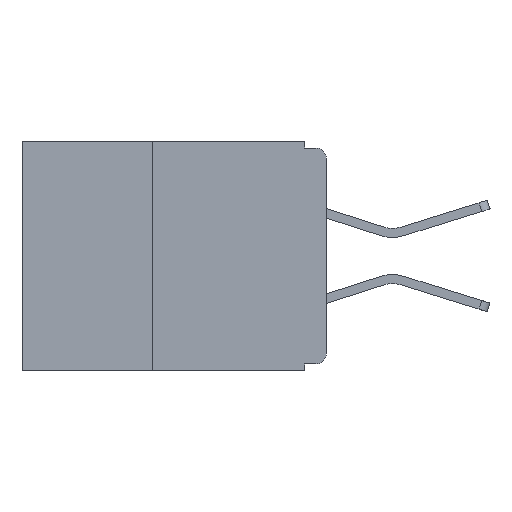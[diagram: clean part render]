
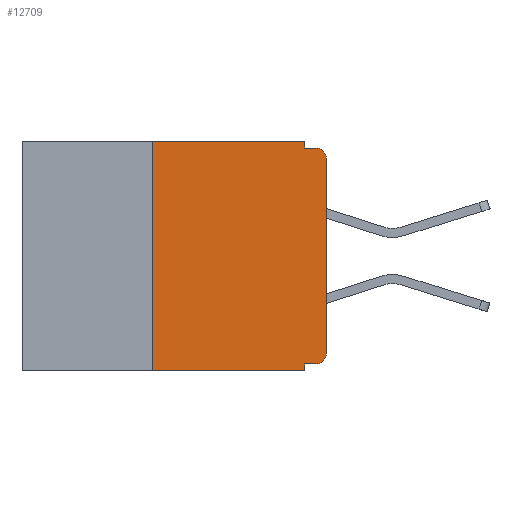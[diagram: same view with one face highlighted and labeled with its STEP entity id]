
A CAD part, left-side view. The second image highlights one B-rep face of the part: STEP entity #12709.
In plain terms, the highlighted planar face has unit normal (-1, 0, 0).
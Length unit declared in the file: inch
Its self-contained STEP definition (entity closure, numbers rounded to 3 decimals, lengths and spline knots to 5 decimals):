
#767 = DIRECTION ( 'NONE',  ( 0., -1., 0. ) ) ;
#1368 = ORIENTED_EDGE ( 'NONE', *, *, #15920, .T. ) ;
#1962 = ORIENTED_EDGE ( 'NONE', *, *, #22748, .T. ) ;
#2030 = LINE ( 'NONE', #27527, #7602 ) ;
#2207 = CARTESIAN_POINT ( 'NONE',  ( 0., 0., -0.305 ) ) ;
#3035 = VERTEX_POINT ( 'NONE', #9136 ) ;
#3124 = VERTEX_POINT ( 'NONE', #2207 ) ;
#3830 = ORIENTED_EDGE ( 'NONE', *, *, #6988, .F. ) ;
#3945 = CARTESIAN_POINT ( 'NONE',  ( 0., 0.031, 0. ) ) ;
#6203 = CARTESIAN_POINT ( 'NONE',  ( 0., 0.015, -0.025 ) ) ;
#6988 = EDGE_CURVE ( 'NONE', #7017, #12612, #12422, .T. ) ;
#7017 = VERTEX_POINT ( 'NONE', #26400 ) ;
#7403 = CARTESIAN_POINT ( 'NONE',  ( 0., 0., -0.025 ) ) ;
#7602 = VECTOR ( 'NONE', #25388, 39.37008 ) ;
#8556 = DIRECTION ( 'NONE',  ( 0., 0., -1. ) ) ;
#8704 = DIRECTION ( 'NONE',  ( 0., 0., -1. ) ) ;
#9136 = CARTESIAN_POINT ( 'NONE',  ( 0., 0.25, -0.33 ) ) ;
#9165 = DIRECTION ( 'NONE',  ( 0., -1., 0. ) ) ;
#9817 = CIRCLE ( 'NONE', #23273, 0.015 ) ;
#10277 = CARTESIAN_POINT ( 'NONE',  ( 0., 0.437, -0.33 ) ) ;
#10391 = CARTESIAN_POINT ( 'NONE',  ( 0., 0.031, -0.32 ) ) ;
#10599 = VERTEX_POINT ( 'NONE', #28992 ) ;
#10800 = CARTESIAN_POINT ( 'NONE',  ( 0., 0.25, -0.33 ) ) ;
#10866 = DIRECTION ( 'NONE',  ( 0., -1., 0. ) ) ;
#10928 = AXIS2_PLACEMENT_3D ( 'NONE', #6203, #22020, #8556 ) ;
#11355 = EDGE_CURVE ( 'NONE', #7017, #3124, #9817, .T. ) ;
#11557 = LINE ( 'NONE', #10800, #12267 ) ;
#11936 = LINE ( 'NONE', #29159, #28253 ) ;
#12267 = VECTOR ( 'NONE', #22029, 39.37008 ) ;
#12422 = LINE ( 'NONE', #27696, #29430 ) ;
#12612 = VERTEX_POINT ( 'NONE', #10391 ) ;
#12709 = ADVANCED_FACE ( 'NONE', ( #18882 ), #17483, .F. ) ;
#12977 = CARTESIAN_POINT ( 'NONE',  ( 0., 0.031, -0.33 ) ) ;
#13052 = CARTESIAN_POINT ( 'NONE',  ( 0., 0.437, 0. ) ) ;
#14250 = VECTOR ( 'NONE', #8704, 39.37008 ) ;
#15321 = DIRECTION ( 'NONE',  ( 0., 0., -1. ) ) ;
#15920 = EDGE_CURVE ( 'NONE', #3035, #28485, #28684, .T. ) ;
#16948 = VECTOR ( 'NONE', #767, 39.37008 ) ;
#17221 = ORIENTED_EDGE ( 'NONE', *, *, #20737, .F. ) ;
#17483 = PLANE ( 'NONE',  #22004 ) ;
#17524 = DIRECTION ( 'NONE',  ( 0., 0., -1. ) ) ;
#17584 = DIRECTION ( 'NONE',  ( -1., 0., 0. ) ) ;
#17616 = CARTESIAN_POINT ( 'NONE',  ( 0., 0.015, -0.305 ) ) ;
#17982 = VECTOR ( 'NONE', #22477, 39.37008 ) ;
#18319 = EDGE_CURVE ( 'NONE', #3035, #19501, #11557, .T. ) ;
#18882 = FACE_OUTER_BOUND ( 'NONE', #23102, .T. ) ;
#19501 = VERTEX_POINT ( 'NONE', #22161 ) ;
#19587 = CARTESIAN_POINT ( 'NONE',  ( 0., 0.031, -0.01 ) ) ;
#20109 = ORIENTED_EDGE ( 'NONE', *, *, #27459, .F. ) ;
#20194 = LINE ( 'NONE', #3945, #14250 ) ;
#20541 = CARTESIAN_POINT ( 'NONE',  ( 0., 0.031, 0. ) ) ;
#20737 = EDGE_CURVE ( 'NONE', #21424, #10599, #28692, .T. ) ;
#21386 = CIRCLE ( 'NONE', #10928, 0.015 ) ;
#21424 = VERTEX_POINT ( 'NONE', #19587 ) ;
#21460 = ORIENTED_EDGE ( 'NONE', *, *, #18319, .F. ) ;
#22004 = AXIS2_PLACEMENT_3D ( 'NONE', #13052, #28577, #15321 ) ;
#22020 = DIRECTION ( 'NONE',  ( -1., 0., 0. ) ) ;
#22029 = DIRECTION ( 'NONE',  ( 0., 0., 1. ) ) ;
#22161 = CARTESIAN_POINT ( 'NONE',  ( 0., 0.25, 0. ) ) ;
#22477 = DIRECTION ( 'NONE',  ( 0., 0., -1. ) ) ;
#22748 = EDGE_CURVE ( 'NONE', #23613, #10599, #21386, .T. ) ;
#22974 = EDGE_CURVE ( 'NONE', #3124, #23613, #2030, .T. ) ;
#23102 = EDGE_LOOP ( 'NONE', ( #24544, #1962, #17221, #29170, #27273, #21460, #1368, #20109, #3830, #24479 ) ) ;
#23158 = LINE ( 'NONE', #24696, #17982 ) ;
#23273 = AXIS2_PLACEMENT_3D ( 'NONE', #17616, #17584, #17524 ) ;
#23500 = VERTEX_POINT ( 'NONE', #20541 ) ;
#23528 = VECTOR ( 'NONE', #10866, 39.37008 ) ;
#23613 = VERTEX_POINT ( 'NONE', #7403 ) ;
#24479 = ORIENTED_EDGE ( 'NONE', *, *, #11355, .T. ) ;
#24544 = ORIENTED_EDGE ( 'NONE', *, *, #22974, .T. ) ;
#24696 = CARTESIAN_POINT ( 'NONE',  ( 0., 0.031, -0.33 ) ) ;
#25125 = EDGE_CURVE ( 'NONE', #23500, #21424, #20194, .T. ) ;
#25388 = DIRECTION ( 'NONE',  ( 0., 0., 1. ) ) ;
#26400 = CARTESIAN_POINT ( 'NONE',  ( 0., 0.015, -0.32 ) ) ;
#26430 = CARTESIAN_POINT ( 'NONE',  ( 0., 0., -0.01 ) ) ;
#27273 = ORIENTED_EDGE ( 'NONE', *, *, #28710, .F. ) ;
#27458 = DIRECTION ( 'NONE',  ( 0., 1., 0. ) ) ;
#27459 = EDGE_CURVE ( 'NONE', #12612, #28485, #23158, .T. ) ;
#27527 = CARTESIAN_POINT ( 'NONE',  ( 0., 0., 0. ) ) ;
#27696 = CARTESIAN_POINT ( 'NONE',  ( 0., 0., -0.32 ) ) ;
#28253 = VECTOR ( 'NONE', #9165, 39.37008 ) ;
#28485 = VERTEX_POINT ( 'NONE', #12977 ) ;
#28577 = DIRECTION ( 'NONE',  ( 1., 0., 0. ) ) ;
#28684 = LINE ( 'NONE', #10277, #16948 ) ;
#28692 = LINE ( 'NONE', #26430, #23528 ) ;
#28710 = EDGE_CURVE ( 'NONE', #19501, #23500, #11936, .T. ) ;
#28992 = CARTESIAN_POINT ( 'NONE',  ( 0., 0.015, -0.01 ) ) ;
#29159 = CARTESIAN_POINT ( 'NONE',  ( 0., 0.437, 0. ) ) ;
#29170 = ORIENTED_EDGE ( 'NONE', *, *, #25125, .F. ) ;
#29430 = VECTOR ( 'NONE', #27458, 39.37008 ) ;
